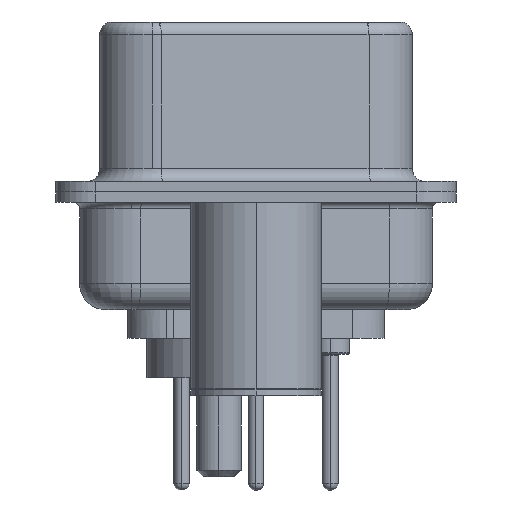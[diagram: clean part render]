
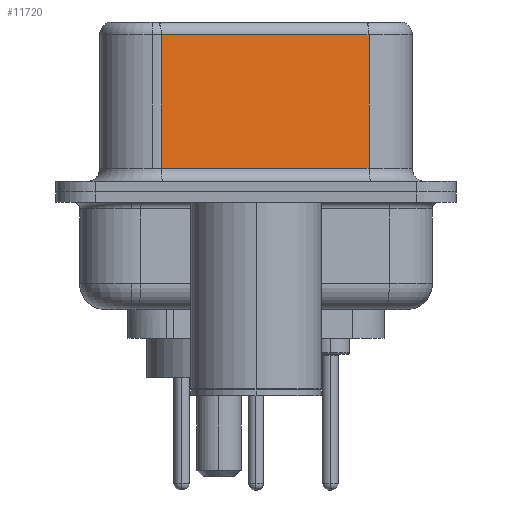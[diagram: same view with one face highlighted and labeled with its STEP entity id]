
A CAD part, left-side view. The second image highlights one B-rep face of the part: STEP entity #11720.
In plain terms, the highlighted planar face has unit normal (-0.985, -0.174, 0).
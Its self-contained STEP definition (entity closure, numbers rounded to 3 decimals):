
#360 = LINE ( 'NONE', #10121, #26732 ) ;
#832 = VECTOR ( 'NONE', #2756, 1000. ) ;
#1486 = CARTESIAN_POINT ( 'NONE',  ( 5.132, -4.322, 6.52 ) ) ;
#2710 = DIRECTION ( 'NONE',  ( 0.985, 0.174, 0. ) ) ;
#2756 = DIRECTION ( 'NONE',  ( 0., 0., -1. ) ) ;
#2997 = ORIENTED_EDGE ( 'NONE', *, *, #6637, .T. ) ;
#3550 = EDGE_CURVE ( 'NONE', #21727, #25437, #13959, .T. ) ;
#4406 = VERTEX_POINT ( 'NONE', #24672 ) ;
#6637 = EDGE_CURVE ( 'NONE', #6948, #4406, #16330, .T. ) ;
#6948 = VERTEX_POINT ( 'NONE', #14292 ) ;
#8569 = DIRECTION ( 'NONE',  ( 0.174, -0.985, 0. ) ) ;
#9207 = CARTESIAN_POINT ( 'NONE',  ( 3.73, 3.628, 6.52 ) ) ;
#9966 = LINE ( 'NONE', #22967, #14819 ) ;
#9991 = CARTESIAN_POINT ( 'NONE',  ( 5.132, -4.322, 0.9 ) ) ;
#10121 = CARTESIAN_POINT ( 'NONE',  ( 5.132, -4.322, 6.02 ) ) ;
#10250 = ORIENTED_EDGE ( 'NONE', *, *, #24824, .T. ) ;
#11294 = FACE_OUTER_BOUND ( 'NONE', #17735, .T. ) ;
#11720 = ADVANCED_FACE ( 'NONE', ( #11294 ), #19319, .F. ) ;
#12340 = DIRECTION ( 'NONE',  ( -0.174, 0.985, 0. ) ) ;
#13312 = VECTOR ( 'NONE', #19408, 1000. ) ;
#13959 = LINE ( 'NONE', #1486, #13312 ) ;
#14292 = CARTESIAN_POINT ( 'NONE',  ( 3.73, 3.628, 6.02 ) ) ;
#14819 = VECTOR ( 'NONE', #8569, 1000. ) ;
#15264 = CARTESIAN_POINT ( 'NONE',  ( 5.132, -4.322, 6.02 ) ) ;
#16330 = LINE ( 'NONE', #9207, #832 ) ;
#17320 = DIRECTION ( 'NONE',  ( -0.174, 0.985, 0. ) ) ;
#17735 = EDGE_LOOP ( 'NONE', ( #25898, #10250, #2997, #26370 ) ) ;
#18646 = AXIS2_PLACEMENT_3D ( 'NONE', #25455, #2710, #17320 ) ;
#19319 = PLANE ( 'NONE',  #18646 ) ;
#19408 = DIRECTION ( 'NONE',  ( 0., 0., -1. ) ) ;
#19926 = EDGE_CURVE ( 'NONE', #4406, #25437, #9966, .T. ) ;
#21727 = VERTEX_POINT ( 'NONE', #15264 ) ;
#22967 = CARTESIAN_POINT ( 'NONE',  ( 5.132, -4.322, 0.9 ) ) ;
#24672 = CARTESIAN_POINT ( 'NONE',  ( 3.73, 3.628, 0.9 ) ) ;
#24824 = EDGE_CURVE ( 'NONE', #21727, #6948, #360, .T. ) ;
#25437 = VERTEX_POINT ( 'NONE', #9991 ) ;
#25455 = CARTESIAN_POINT ( 'NONE',  ( 5.132, -4.322, 6.52 ) ) ;
#25898 = ORIENTED_EDGE ( 'NONE', *, *, #3550, .F. ) ;
#26370 = ORIENTED_EDGE ( 'NONE', *, *, #19926, .T. ) ;
#26732 = VECTOR ( 'NONE', #12340, 1000. ) ;
